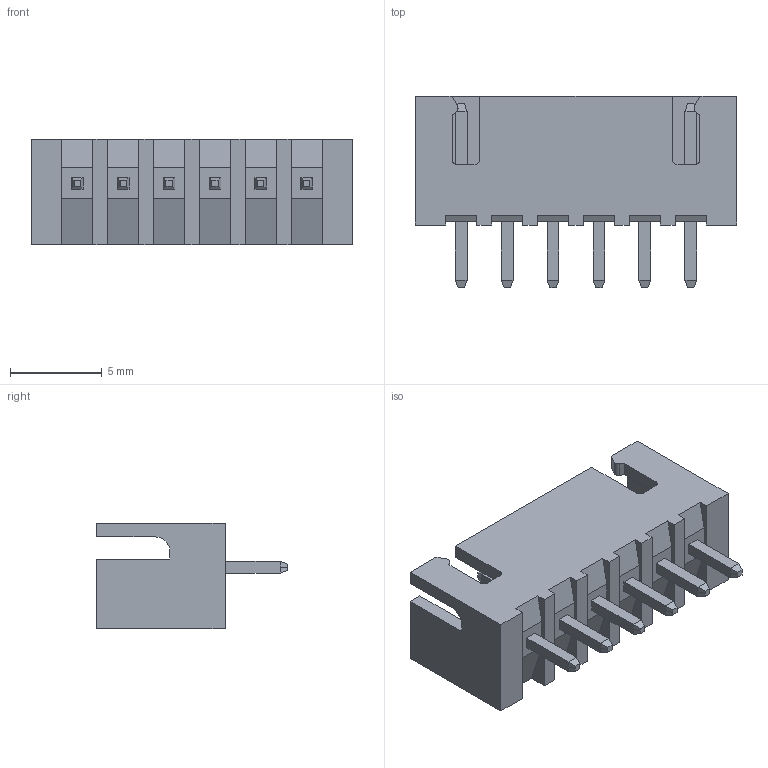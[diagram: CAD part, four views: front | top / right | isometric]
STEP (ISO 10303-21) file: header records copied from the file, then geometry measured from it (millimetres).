
FILE_DESCRIPTION (( 'STEP AP203' ), '1' );
FILE_NAME ('14K-506-415-AA1.STEP', '2024-02-23T16:29:34', ( '' ), ( '' ), 'SwSTEP 2.0', 'SolidWorks 2023', '' );
FILE_SCHEMA (( 'CONFIG_CONTROL_DESIGN' ));
Length unit declared in the file: millimetre
Products named in the file (3): 14K Series Pin Header Insulator_506; 14K Series Pin_15; 14K-506-415-AA1
Assembly tree (7 placements, depth 2):
  14K-506-415-AA1
    14K Series Pin Header Insulator_506
    14K Series Pin_15  x6
Bounding box: 17.5 x 10.4 x 5.75 mm (x, y, z)
Volume: 332.9 mm3; surface area: 910.6 mm2
Topology: 7 solids, 7 shells, 196 faces, 498 edges, 316 vertices
Faces by surface type: plane 187, cylinder 9
Entity records: 4175 total; most frequent: CARTESIAN_POINT 670, ORIENTED_EDGE 656, DIRECTION 598, EDGE_CURVE 328, VECTOR 310, LINE 310, VERTEX_POINT 216, AXIS2_PLACEMENT_3D 144
